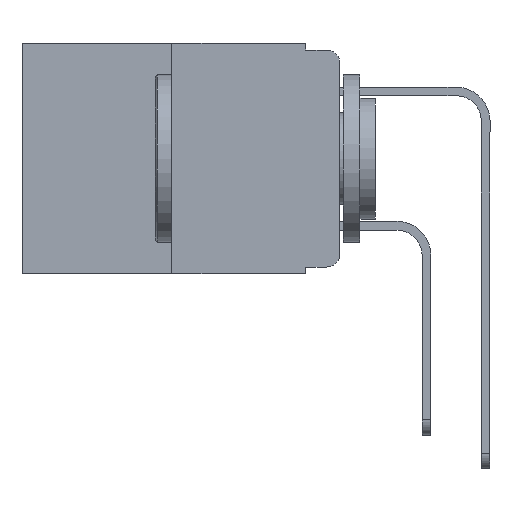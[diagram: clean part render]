
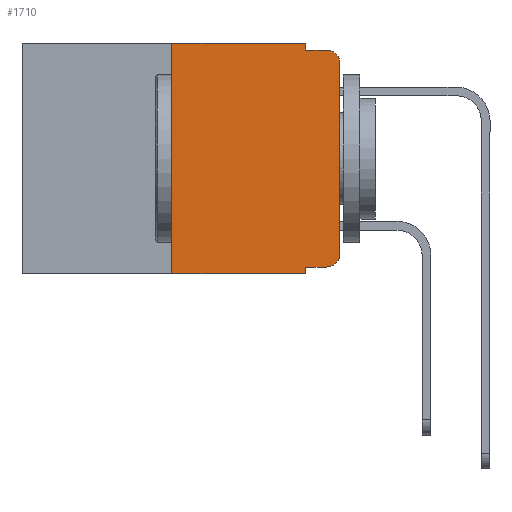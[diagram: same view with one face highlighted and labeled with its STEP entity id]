
A CAD part, left-side view. The second image highlights one B-rep face of the part: STEP entity #1710.
In plain terms, the highlighted planar face has unit normal (-1, 0, 0).
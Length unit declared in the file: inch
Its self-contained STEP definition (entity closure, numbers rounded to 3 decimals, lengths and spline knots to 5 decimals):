
#360 = EDGE_CURVE ( 'NONE', #1192, #15010, #6833, .T. ) ;
#585 = DIRECTION ( 'NONE',  ( 0., 0., 1. ) ) ;
#615 = CARTESIAN_POINT ( 'NONE',  ( 0., 0.02, -0.313 ) ) ;
#973 = CARTESIAN_POINT ( 'NONE',  ( 0., 0.051, 0. ) ) ;
#1192 = VERTEX_POINT ( 'NONE', #14607 ) ;
#1243 = ORIENTED_EDGE ( 'NONE', *, *, #10727, .F. ) ;
#1244 = EDGE_CURVE ( 'NONE', #10622, #1693, #8610, .T. ) ;
#1638 = VERTEX_POINT ( 'NONE', #2726 ) ;
#1677 = AXIS2_PLACEMENT_3D ( 'NONE', #615, #9338, #1928 ) ;
#1693 = VERTEX_POINT ( 'NONE', #4304 ) ;
#1710 = ADVANCED_FACE ( 'NONE', ( #11706 ), #4329, .F. ) ;
#1808 = VERTEX_POINT ( 'NONE', #5101 ) ;
#1928 = DIRECTION ( 'NONE',  ( 0., 0., -1. ) ) ;
#2075 = LINE ( 'NONE', #14534, #11407 ) ;
#2107 = EDGE_CURVE ( 'NONE', #1693, #13164, #4538, .T. ) ;
#2187 = CARTESIAN_POINT ( 'NONE',  ( 0., 0.051, 0. ) ) ;
#2433 = CARTESIAN_POINT ( 'NONE',  ( 0., 0.473, -0.343 ) ) ;
#2558 = CARTESIAN_POINT ( 'NONE',  ( 0., 0.473, 0. ) ) ;
#2726 = CARTESIAN_POINT ( 'NONE',  ( 0., 0., -0.03 ) ) ;
#2840 = ORIENTED_EDGE ( 'NONE', *, *, #12180, .T. ) ;
#3126 = DIRECTION ( 'NONE',  ( 0., -1., 0. ) ) ;
#3241 = CIRCLE ( 'NONE', #1677, 0.02 ) ;
#3422 = ORIENTED_EDGE ( 'NONE', *, *, #6292, .T. ) ;
#3500 = CARTESIAN_POINT ( 'NONE',  ( 0., 0., -0.313 ) ) ;
#3520 = VECTOR ( 'NONE', #585, 39.37008 ) ;
#3613 = VERTEX_POINT ( 'NONE', #3500 ) ;
#3693 = AXIS2_PLACEMENT_3D ( 'NONE', #2558, #4535, #4496 ) ;
#3891 = LINE ( 'NONE', #2433, #4283 ) ;
#4211 = ORIENTED_EDGE ( 'NONE', *, *, #1244, .F. ) ;
#4283 = VECTOR ( 'NONE', #10967, 39.37008 ) ;
#4304 = CARTESIAN_POINT ( 'NONE',  ( 0., 0.051, -0.01 ) ) ;
#4329 = PLANE ( 'NONE',  #3693 ) ;
#4496 = DIRECTION ( 'NONE',  ( 0., 0., -1. ) ) ;
#4535 = DIRECTION ( 'NONE',  ( 1., 0., 0. ) ) ;
#4538 = LINE ( 'NONE', #8581, #10612 ) ;
#4669 = DIRECTION ( 'NONE',  ( 0., 0., -1. ) ) ;
#4785 = DIRECTION ( 'NONE',  ( 0., 0., -1. ) ) ;
#4833 = EDGE_CURVE ( 'NONE', #1192, #1808, #3891, .T. ) ;
#4983 = CARTESIAN_POINT ( 'NONE',  ( 0., 0.473, 0. ) ) ;
#5101 = CARTESIAN_POINT ( 'NONE',  ( 0., 0.051, -0.343 ) ) ;
#5155 = VERTEX_POINT ( 'NONE', #11466 ) ;
#5463 = EDGE_CURVE ( 'NONE', #1638, #13164, #9250, .T. ) ;
#5846 = VECTOR ( 'NONE', #12183, 39.37008 ) ;
#6292 = EDGE_CURVE ( 'NONE', #3613, #1638, #2075, .T. ) ;
#6610 = VERTEX_POINT ( 'NONE', #11574 ) ;
#6833 = LINE ( 'NONE', #15557, #3520 ) ;
#7056 = CARTESIAN_POINT ( 'NONE',  ( 0., 0.051, -0.333 ) ) ;
#7229 = DIRECTION ( 'NONE',  ( -1., 0., 0. ) ) ;
#7869 = ORIENTED_EDGE ( 'NONE', *, *, #360, .F. ) ;
#8529 = LINE ( 'NONE', #13155, #8909 ) ;
#8581 = CARTESIAN_POINT ( 'NONE',  ( 0., 0.051, -0.01 ) ) ;
#8610 = LINE ( 'NONE', #2187, #14451 ) ;
#8905 = LINE ( 'NONE', #7056, #15450 ) ;
#8909 = VECTOR ( 'NONE', #4785, 39.37008 ) ;
#9250 = CIRCLE ( 'NONE', #9890, 0.02 ) ;
#9338 = DIRECTION ( 'NONE',  ( -1., 0., 0. ) ) ;
#9890 = AXIS2_PLACEMENT_3D ( 'NONE', #14257, #7229, #15414 ) ;
#9915 = CARTESIAN_POINT ( 'NONE',  ( 0., 0.25, 0. ) ) ;
#10288 = ORIENTED_EDGE ( 'NONE', *, *, #2107, .F. ) ;
#10612 = VECTOR ( 'NONE', #3126, 39.37008 ) ;
#10618 = EDGE_LOOP ( 'NONE', ( #3422, #13028, #10288, #4211, #1243, #7869, #14474, #14837, #15210, #2840 ) ) ;
#10622 = VERTEX_POINT ( 'NONE', #973 ) ;
#10727 = EDGE_CURVE ( 'NONE', #15010, #10622, #15266, .T. ) ;
#10967 = DIRECTION ( 'NONE',  ( 0., -1., 0. ) ) ;
#11407 = VECTOR ( 'NONE', #12267, 39.37008 ) ;
#11466 = CARTESIAN_POINT ( 'NONE',  ( 0., 0.051, -0.333 ) ) ;
#11574 = CARTESIAN_POINT ( 'NONE',  ( 0., 0.02, -0.333 ) ) ;
#11706 = FACE_OUTER_BOUND ( 'NONE', #10618, .T. ) ;
#11798 = DIRECTION ( 'NONE',  ( 0., -1., 0. ) ) ;
#12180 = EDGE_CURVE ( 'NONE', #6610, #3613, #3241, .T. ) ;
#12183 = DIRECTION ( 'NONE',  ( 0., -1., 0. ) ) ;
#12217 = CARTESIAN_POINT ( 'NONE',  ( 0., 0.02, -0.01 ) ) ;
#12267 = DIRECTION ( 'NONE',  ( 0., 0., 1. ) ) ;
#12959 = EDGE_CURVE ( 'NONE', #5155, #6610, #8905, .T. ) ;
#13028 = ORIENTED_EDGE ( 'NONE', *, *, #5463, .T. ) ;
#13155 = CARTESIAN_POINT ( 'NONE',  ( 0., 0.051, 0. ) ) ;
#13164 = VERTEX_POINT ( 'NONE', #12217 ) ;
#13721 = EDGE_CURVE ( 'NONE', #5155, #1808, #8529, .T. ) ;
#14257 = CARTESIAN_POINT ( 'NONE',  ( 0., 0.02, -0.03 ) ) ;
#14451 = VECTOR ( 'NONE', #4669, 39.37008 ) ;
#14474 = ORIENTED_EDGE ( 'NONE', *, *, #4833, .T. ) ;
#14534 = CARTESIAN_POINT ( 'NONE',  ( 0., 0., 0. ) ) ;
#14607 = CARTESIAN_POINT ( 'NONE',  ( 0., 0.25, -0.343 ) ) ;
#14837 = ORIENTED_EDGE ( 'NONE', *, *, #13721, .F. ) ;
#15010 = VERTEX_POINT ( 'NONE', #9915 ) ;
#15210 = ORIENTED_EDGE ( 'NONE', *, *, #12959, .T. ) ;
#15266 = LINE ( 'NONE', #4983, #5846 ) ;
#15414 = DIRECTION ( 'NONE',  ( 0., 0., -1. ) ) ;
#15450 = VECTOR ( 'NONE', #11798, 39.37008 ) ;
#15557 = CARTESIAN_POINT ( 'NONE',  ( 0., 0.25, 0. ) ) ;
